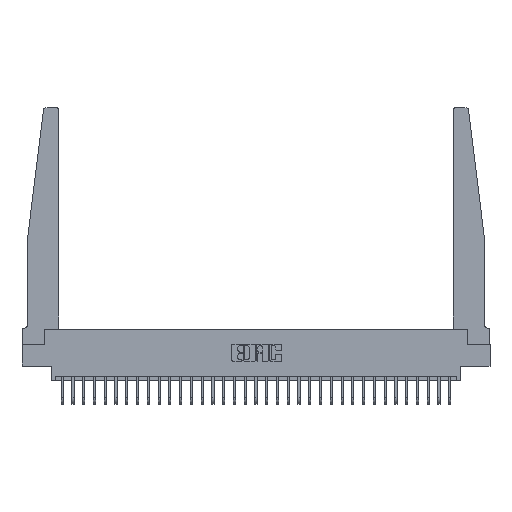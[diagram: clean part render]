
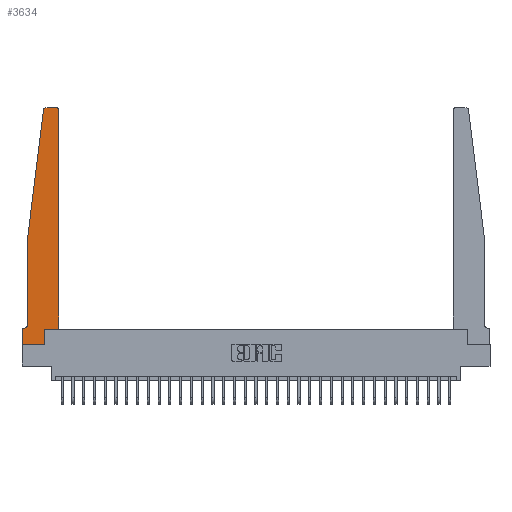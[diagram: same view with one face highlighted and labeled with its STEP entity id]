
A CAD part, top view. The second image highlights one B-rep face of the part: STEP entity #3634.
In plain terms, the highlighted planar face has unit normal (0, 0, 1).
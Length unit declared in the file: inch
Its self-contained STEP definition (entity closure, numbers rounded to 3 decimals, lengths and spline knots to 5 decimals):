
#59 = VECTOR ( 'NONE', #22816, 39.37008 ) ;
#217 = VERTEX_POINT ( 'NONE', #2510 ) ;
#306 = AXIS2_PLACEMENT_3D ( 'NONE', #20445, #7191, #22641 ) ;
#568 = CARTESIAN_POINT ( 'NONE',  ( 0.395, 2.75, 0.37 ) ) ;
#581 = CARTESIAN_POINT ( 'NONE',  ( 0.065, 0.1875, 0.37 ) ) ;
#1614 = EDGE_CURVE ( 'NONE', #8737, #7975, #17787, .T. ) ;
#1663 = PLANE ( 'NONE',  #26677 ) ;
#1957 = CARTESIAN_POINT ( 'NONE',  ( 0.015, 0.2375, 0.37 ) ) ;
#2372 = VERTEX_POINT ( 'NONE', #25580 ) ;
#2452 = CIRCLE ( 'NONE', #306, 0.03 ) ;
#2510 = CARTESIAN_POINT ( 'NONE',  ( 0.24675, 2.72367, 0.37 ) ) ;
#3416 = CARTESIAN_POINT ( 'NONE',  ( 0.25, 2.75, 0.37 ) ) ;
#3535 = ORIENTED_EDGE ( 'NONE', *, *, #24254, .T. ) ;
#3634 = ADVANCED_FACE ( 'NONE', ( #14936 ), #1663, .T. ) ;
#3659 = VERTEX_POINT ( 'NONE', #4001 ) ;
#3865 = CARTESIAN_POINT ( 'NONE',  ( 0.425, 0.18, 0.37 ) ) ;
#4001 = CARTESIAN_POINT ( 'NONE',  ( 0.425, 0.18, 0.37 ) ) ;
#4106 = VECTOR ( 'NONE', #10286, 39.37008 ) ;
#4160 = DIRECTION ( 'NONE',  ( 0., 0., 1. ) ) ;
#4198 = DIRECTION ( 'NONE',  ( -1., 0., 0. ) ) ;
#4523 = LINE ( 'NONE', #5445, #15569 ) ;
#4814 = LINE ( 'NONE', #9585, #28316 ) ;
#5058 = DIRECTION ( 'NONE',  ( -1., 0., 0. ) ) ;
#5445 = CARTESIAN_POINT ( 'NONE',  ( 0.425, 0.18, 0.37 ) ) ;
#5677 = EDGE_CURVE ( 'NONE', #13092, #28377, #21718, .T. ) ;
#5756 = ORIENTED_EDGE ( 'NONE', *, *, #13340, .T. ) ;
#6123 = DIRECTION ( 'NONE',  ( 0., 0., 1. ) ) ;
#6498 = VECTOR ( 'NONE', #15013, 39.37008 ) ;
#6781 = CIRCLE ( 'NONE', #21050, 0.05 ) ;
#6984 = CARTESIAN_POINT ( 'NONE',  ( 0., 0.1875, 0.37 ) ) ;
#7191 = DIRECTION ( 'NONE',  ( 0., 0., 1. ) ) ;
#7660 = DIRECTION ( 'NONE',  ( 1., 0., 0. ) ) ;
#7944 = ORIENTED_EDGE ( 'NONE', *, *, #5677, .T. ) ;
#7975 = VERTEX_POINT ( 'NONE', #6984 ) ;
#8311 = ORIENTED_EDGE ( 'NONE', *, *, #26964, .T. ) ;
#8528 = VERTEX_POINT ( 'NONE', #568 ) ;
#8537 = ORIENTED_EDGE ( 'NONE', *, *, #17760, .T. ) ;
#8675 = VECTOR ( 'NONE', #21093, 39.37008 ) ;
#8737 = VERTEX_POINT ( 'NONE', #21263 ) ;
#9585 = CARTESIAN_POINT ( 'NONE',  ( 0., 0., 0.37 ) ) ;
#9603 = VERTEX_POINT ( 'NONE', #17047 ) ;
#10130 = ORIENTED_EDGE ( 'NONE', *, *, #17099, .T. ) ;
#10286 = DIRECTION ( 'NONE',  ( 0., -1., 0. ) ) ;
#10473 = CARTESIAN_POINT ( 'NONE',  ( 0., 0.1875, 0.37 ) ) ;
#11165 = ORIENTED_EDGE ( 'NONE', *, *, #25958, .T. ) ;
#11765 = LINE ( 'NONE', #27284, #59 ) ;
#12369 = VERTEX_POINT ( 'NONE', #22624 ) ;
#12623 = EDGE_CURVE ( 'NONE', #7975, #2372, #23429, .T. ) ;
#12781 = CARTESIAN_POINT ( 'NONE',  ( 0., 0., 0.37 ) ) ;
#13092 = VERTEX_POINT ( 'NONE', #25288 ) ;
#13340 = EDGE_CURVE ( 'NONE', #12369, #217, #13376, .T. ) ;
#13376 = CIRCLE ( 'NONE', #15285, 0.03 ) ;
#13984 = DIRECTION ( 'NONE',  ( 1., 0., 0. ) ) ;
#13994 = CARTESIAN_POINT ( 'NONE',  ( 0.425, 2.72, 0.37 ) ) ;
#14490 = EDGE_CURVE ( 'NONE', #28377, #8737, #6781, .T. ) ;
#14936 = FACE_OUTER_BOUND ( 'NONE', #22106, .T. ) ;
#15013 = DIRECTION ( 'NONE',  ( 0., -1., 0. ) ) ;
#15285 = AXIS2_PLACEMENT_3D ( 'NONE', #17371, #4160, #19619 ) ;
#15401 = ORIENTED_EDGE ( 'NONE', *, *, #1614, .T. ) ;
#15569 = VECTOR ( 'NONE', #7660, 39.37008 ) ;
#15589 = ORIENTED_EDGE ( 'NONE', *, *, #16670, .T. ) ;
#16450 = ORIENTED_EDGE ( 'NONE', *, *, #12623, .T. ) ;
#16613 = ORIENTED_EDGE ( 'NONE', *, *, #14490, .T. ) ;
#16670 = EDGE_CURVE ( 'NONE', #20088, #9603, #25276, .T. ) ;
#17047 = CARTESIAN_POINT ( 'NONE',  ( 0.2605, 0.18, 0.37 ) ) ;
#17099 = EDGE_CURVE ( 'NONE', #22588, #8528, #2452, .T. ) ;
#17107 = VECTOR ( 'NONE', #5058, 39.37008 ) ;
#17371 = CARTESIAN_POINT ( 'NONE',  ( 0.27653, 2.72, 0.37 ) ) ;
#17405 = DIRECTION ( 'NONE',  ( 0., 0., -1. ) ) ;
#17760 = EDGE_CURVE ( 'NONE', #8528, #12369, #26975, .T. ) ;
#17787 = LINE ( 'NONE', #581, #17107 ) ;
#18253 = CARTESIAN_POINT ( 'NONE',  ( 0.065, 0.2375, 0.37 ) ) ;
#19041 = CARTESIAN_POINT ( 'NONE',  ( 0.2605, 0.18, 0.37 ) ) ;
#19619 = DIRECTION ( 'NONE',  ( 1., 0., 0. ) ) ;
#20088 = VERTEX_POINT ( 'NONE', #25540 ) ;
#20445 = CARTESIAN_POINT ( 'NONE',  ( 0.395, 2.72, 0.37 ) ) ;
#21050 = AXIS2_PLACEMENT_3D ( 'NONE', #1957, #17405, #4198 ) ;
#21093 = DIRECTION ( 'NONE',  ( -1., 0., 0. ) ) ;
#21263 = CARTESIAN_POINT ( 'NONE',  ( 0.015, 0.1875, 0.37 ) ) ;
#21570 = DIRECTION ( 'NONE',  ( 1., 0., 0. ) ) ;
#21718 = LINE ( 'NONE', #23488, #4106 ) ;
#22073 = LINE ( 'NONE', #3865, #27268 ) ;
#22106 = EDGE_LOOP ( 'NONE', ( #8537, #5756, #11165, #7944, #16613, #15401, #16450, #27868, #15589, #3535, #8311, #10130 ) ) ;
#22588 = VERTEX_POINT ( 'NONE', #13994 ) ;
#22624 = CARTESIAN_POINT ( 'NONE',  ( 0.27653, 2.75, 0.37 ) ) ;
#22641 = DIRECTION ( 'NONE',  ( 1., 0., 0. ) ) ;
#22816 = DIRECTION ( 'NONE',  ( -0.122, -0.992, 0. ) ) ;
#23429 = LINE ( 'NONE', #12781, #6498 ) ;
#23464 = DIRECTION ( 'NONE',  ( 0., 1., 0. ) ) ;
#23488 = CARTESIAN_POINT ( 'NONE',  ( 0.065, 1.25, 0.37 ) ) ;
#24254 = EDGE_CURVE ( 'NONE', #9603, #3659, #4523, .T. ) ;
#24577 = VECTOR ( 'NONE', #23464, 39.37008 ) ;
#25276 = LINE ( 'NONE', #19041, #24577 ) ;
#25288 = CARTESIAN_POINT ( 'NONE',  ( 0.065, 1.25, 0.37 ) ) ;
#25540 = CARTESIAN_POINT ( 'NONE',  ( 0.2605, 0., 0.37 ) ) ;
#25580 = CARTESIAN_POINT ( 'NONE',  ( 0., 0., 0.37 ) ) ;
#25958 = EDGE_CURVE ( 'NONE', #217, #13092, #11765, .T. ) ;
#26677 = AXIS2_PLACEMENT_3D ( 'NONE', #10473, #6123, #21570 ) ;
#26714 = EDGE_CURVE ( 'NONE', #2372, #20088, #4814, .T. ) ;
#26964 = EDGE_CURVE ( 'NONE', #3659, #22588, #22073, .T. ) ;
#26975 = LINE ( 'NONE', #3416, #8675 ) ;
#27268 = VECTOR ( 'NONE', #28283, 39.37008 ) ;
#27284 = CARTESIAN_POINT ( 'NONE',  ( 0.065, 1.25, 0.37 ) ) ;
#27868 = ORIENTED_EDGE ( 'NONE', *, *, #26714, .T. ) ;
#28283 = DIRECTION ( 'NONE',  ( 0., 1., 0. ) ) ;
#28316 = VECTOR ( 'NONE', #13984, 39.37008 ) ;
#28377 = VERTEX_POINT ( 'NONE', #18253 ) ;
